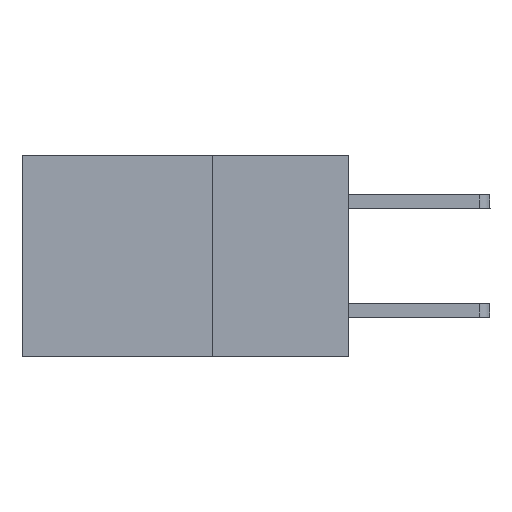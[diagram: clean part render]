
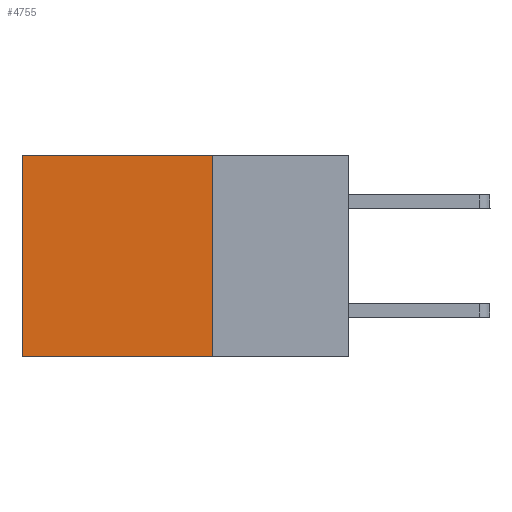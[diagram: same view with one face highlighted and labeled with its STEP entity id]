
A CAD part, left-side view. The second image highlights one B-rep face of the part: STEP entity #4755.
In plain terms, the highlighted planar face has unit normal (-1, 0, 0).
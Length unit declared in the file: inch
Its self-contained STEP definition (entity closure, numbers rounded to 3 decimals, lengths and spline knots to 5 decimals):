
#711 = CARTESIAN_POINT ( 'NONE',  ( 0.298, 0.25, -0.37 ) ) ;
#908 = VERTEX_POINT ( 'NONE', #7947 ) ;
#1080 = CARTESIAN_POINT ( 'NONE',  ( 0.298, 0.25, 0. ) ) ;
#2013 = VECTOR ( 'NONE', #2255, 39.37008 ) ;
#2186 = EDGE_CURVE ( 'NONE', #3955, #908, #4742, .T. ) ;
#2207 = CARTESIAN_POINT ( 'NONE',  ( 0.298, 0.25, 0. ) ) ;
#2255 = DIRECTION ( 'NONE',  ( 0., 1., 0. ) ) ;
#2342 = VECTOR ( 'NONE', #8346, 39.37008 ) ;
#2797 = CARTESIAN_POINT ( 'NONE',  ( 0.298, 0.25, 0. ) ) ;
#3615 = DIRECTION ( 'NONE',  ( 1., 0., 0. ) ) ;
#3955 = VERTEX_POINT ( 'NONE', #2797 ) ;
#4742 = LINE ( 'NONE', #2207, #2013 ) ;
#4755 = ADVANCED_FACE ( 'NONE', ( #5341 ), #9196, .F. ) ;
#5190 = DIRECTION ( 'NONE',  ( 0., 0., -1. ) ) ;
#5278 = EDGE_CURVE ( 'NONE', #908, #7132, #9187, .T. ) ;
#5321 = CARTESIAN_POINT ( 'NONE',  ( 0.298, 0.25, -0.37 ) ) ;
#5341 = FACE_OUTER_BOUND ( 'NONE', #6607, .T. ) ;
#5598 = ORIENTED_EDGE ( 'NONE', *, *, #7978, .F. ) ;
#6361 = AXIS2_PLACEMENT_3D ( 'NONE', #8354, #3615, #5190 ) ;
#6607 = EDGE_LOOP ( 'NONE', ( #8800, #5598, #7907, #7137 ) ) ;
#6790 = DIRECTION ( 'NONE',  ( 0., 0., -1. ) ) ;
#6820 = CARTESIAN_POINT ( 'NONE',  ( 0.298, 0.6, 0. ) ) ;
#7132 = VERTEX_POINT ( 'NONE', #10358 ) ;
#7137 = ORIENTED_EDGE ( 'NONE', *, *, #2186, .T. ) ;
#7422 = VECTOR ( 'NONE', #6790, 39.37008 ) ;
#7907 = ORIENTED_EDGE ( 'NONE', *, *, #9659, .F. ) ;
#7947 = CARTESIAN_POINT ( 'NONE',  ( 0.298, 0.6, 0. ) ) ;
#7978 = EDGE_CURVE ( 'NONE', #8778, #7132, #9368, .T. ) ;
#8346 = DIRECTION ( 'NONE',  ( 0., 0., -1. ) ) ;
#8354 = CARTESIAN_POINT ( 'NONE',  ( 0.298, 0.25, 0. ) ) ;
#8721 = DIRECTION ( 'NONE',  ( 0., 1., 0. ) ) ;
#8778 = VERTEX_POINT ( 'NONE', #5321 ) ;
#8800 = ORIENTED_EDGE ( 'NONE', *, *, #5278, .T. ) ;
#8820 = VECTOR ( 'NONE', #8721, 39.37008 ) ;
#9105 = LINE ( 'NONE', #1080, #7422 ) ;
#9187 = LINE ( 'NONE', #6820, #2342 ) ;
#9196 = PLANE ( 'NONE',  #6361 ) ;
#9368 = LINE ( 'NONE', #711, #8820 ) ;
#9659 = EDGE_CURVE ( 'NONE', #3955, #8778, #9105, .T. ) ;
#10358 = CARTESIAN_POINT ( 'NONE',  ( 0.298, 0.6, -0.37 ) ) ;
